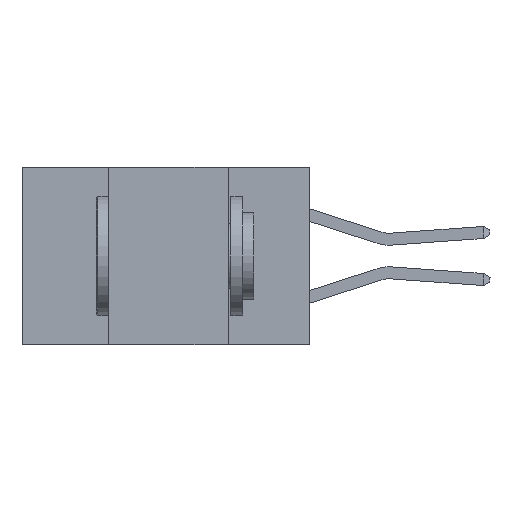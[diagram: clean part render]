
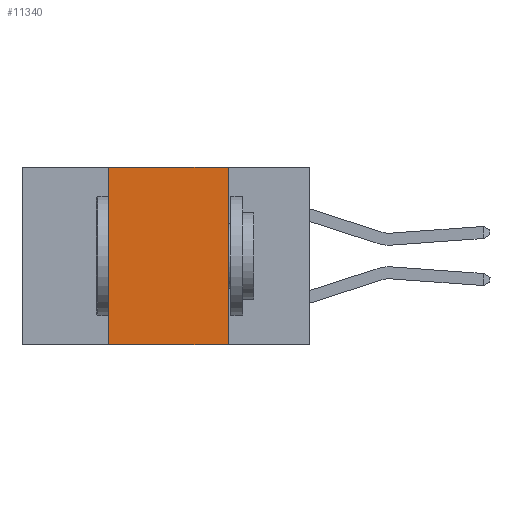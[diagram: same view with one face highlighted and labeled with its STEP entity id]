
A CAD part, left-side view. The second image highlights one B-rep face of the part: STEP entity #11340.
In plain terms, the highlighted planar face has unit normal (-1, 0, 0).
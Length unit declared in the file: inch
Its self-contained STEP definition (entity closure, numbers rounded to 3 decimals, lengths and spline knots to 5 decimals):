
#343 = CARTESIAN_POINT ( 'NONE',  ( 0., 0.42, 0. ) ) ;
#1162 = CARTESIAN_POINT ( 'NONE',  ( 0., 0.6, 0. ) ) ;
#2004 = EDGE_CURVE ( 'NONE', #3374, #10269, #20630, .T. ) ;
#2566 = LINE ( 'NONE', #343, #12264 ) ;
#3374 = VERTEX_POINT ( 'NONE', #14131 ) ;
#5629 = VECTOR ( 'NONE', #21246, 39.37008 ) ;
#6239 = EDGE_CURVE ( 'NONE', #23459, #10269, #8189, .T. ) ;
#8189 = LINE ( 'NONE', #8464, #18821 ) ;
#8319 = CARTESIAN_POINT ( 'NONE',  ( 0., 0.17, 0. ) ) ;
#8464 = CARTESIAN_POINT ( 'NONE',  ( 0., 0.6, -0.37 ) ) ;
#8714 = FACE_OUTER_BOUND ( 'NONE', #9670, .T. ) ;
#8943 = ORIENTED_EDGE ( 'NONE', *, *, #17517, .F. ) ;
#9224 = AXIS2_PLACEMENT_3D ( 'NONE', #17397, #19060, #21219 ) ;
#9670 = EDGE_LOOP ( 'NONE', ( #18201, #8943, #26822, #24780 ) ) ;
#10269 = VERTEX_POINT ( 'NONE', #12222 ) ;
#11340 = ADVANCED_FACE ( 'NONE', ( #8714 ), #15140, .F. ) ;
#12222 = CARTESIAN_POINT ( 'NONE',  ( 0., 0.17, -0.37 ) ) ;
#12264 = VECTOR ( 'NONE', #12944, 39.37008 ) ;
#12790 = VECTOR ( 'NONE', #26785, 39.37008 ) ;
#12944 = DIRECTION ( 'NONE',  ( 0., 0., 1. ) ) ;
#13108 = LINE ( 'NONE', #1162, #12790 ) ;
#14131 = CARTESIAN_POINT ( 'NONE',  ( 0., 0.17, 0. ) ) ;
#15140 = PLANE ( 'NONE',  #9224 ) ;
#17397 = CARTESIAN_POINT ( 'NONE',  ( 0., 0.6, 0. ) ) ;
#17517 = EDGE_CURVE ( 'NONE', #20753, #3374, #13108, .T. ) ;
#17573 = CARTESIAN_POINT ( 'NONE',  ( 0., 0.42, -0.37 ) ) ;
#18201 = ORIENTED_EDGE ( 'NONE', *, *, #2004, .F. ) ;
#18821 = VECTOR ( 'NONE', #20750, 39.37008 ) ;
#19060 = DIRECTION ( 'NONE',  ( 1., 0., 0. ) ) ;
#19198 = CARTESIAN_POINT ( 'NONE',  ( 0., 0.42, 0. ) ) ;
#20630 = LINE ( 'NONE', #8319, #5629 ) ;
#20750 = DIRECTION ( 'NONE',  ( 0., -1., 0. ) ) ;
#20753 = VERTEX_POINT ( 'NONE', #19198 ) ;
#21219 = DIRECTION ( 'NONE',  ( 0., 0., -1. ) ) ;
#21246 = DIRECTION ( 'NONE',  ( 0., 0., -1. ) ) ;
#23459 = VERTEX_POINT ( 'NONE', #17573 ) ;
#24780 = ORIENTED_EDGE ( 'NONE', *, *, #6239, .T. ) ;
#26785 = DIRECTION ( 'NONE',  ( 0., -1., 0. ) ) ;
#26822 = ORIENTED_EDGE ( 'NONE', *, *, #26849, .F. ) ;
#26849 = EDGE_CURVE ( 'NONE', #23459, #20753, #2566, .T. ) ;
